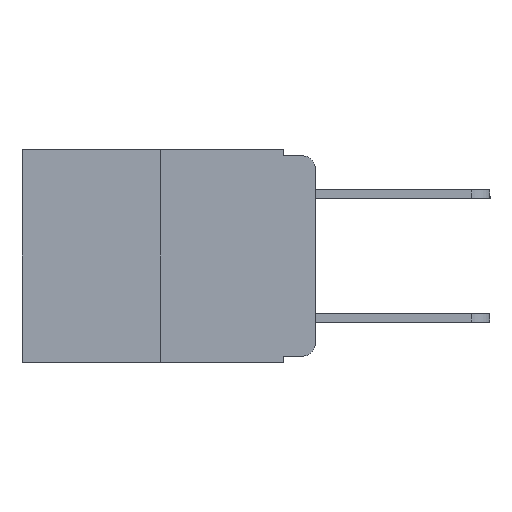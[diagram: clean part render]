
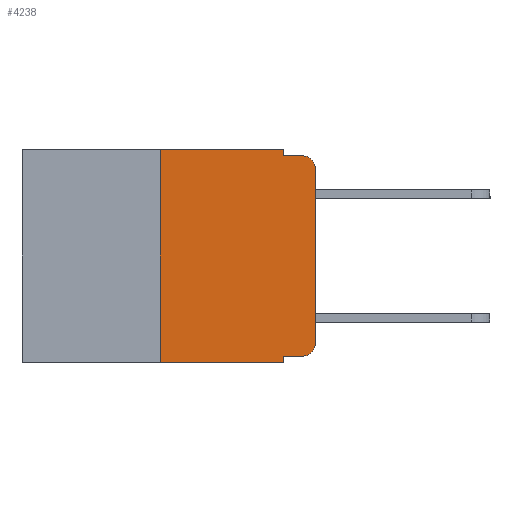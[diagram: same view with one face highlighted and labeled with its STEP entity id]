
A CAD part, left-side view. The second image highlights one B-rep face of the part: STEP entity #4238.
In plain terms, the highlighted planar face has unit normal (-1, 0, 0).
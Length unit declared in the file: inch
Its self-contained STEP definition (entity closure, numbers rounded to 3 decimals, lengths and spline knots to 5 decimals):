
#136 = CIRCLE ( 'NONE', #7155, 0.02 ) ;
#248 = PLANE ( 'NONE',  #5936 ) ;
#509 = EDGE_CURVE ( 'NONE', #4384, #8145, #9554, .T. ) ;
#540 = VECTOR ( 'NONE', #5048, 39.37008 ) ;
#561 = FACE_OUTER_BOUND ( 'NONE', #1097, .T. ) ;
#626 = VERTEX_POINT ( 'NONE', #2970 ) ;
#870 = LINE ( 'NONE', #10910, #10243 ) ;
#949 = DIRECTION ( 'NONE',  ( 0., -1., 0. ) ) ;
#1097 = EDGE_LOOP ( 'NONE', ( #1823, #5097, #2701, #4513, #5716, #2950, #6940, #9742, #6254, #6052 ) ) ;
#1120 = CARTESIAN_POINT ( 'NONE',  ( 0., 0.051, -0.343 ) ) ;
#1334 = EDGE_CURVE ( 'NONE', #10376, #5149, #3584, .T. ) ;
#1509 = DIRECTION ( 'NONE',  ( 1., 0., 0. ) ) ;
#1540 = DIRECTION ( 'NONE',  ( 0., -1., 0. ) ) ;
#1544 = CARTESIAN_POINT ( 'NONE',  ( 0., 0.02, -0.313 ) ) ;
#1609 = VERTEX_POINT ( 'NONE', #5969 ) ;
#1823 = ORIENTED_EDGE ( 'NONE', *, *, #4086, .T. ) ;
#1967 = EDGE_CURVE ( 'NONE', #5149, #4384, #870, .T. ) ;
#2313 = VERTEX_POINT ( 'NONE', #8914 ) ;
#2659 = DIRECTION ( 'NONE',  ( 0., 0., -1. ) ) ;
#2701 = ORIENTED_EDGE ( 'NONE', *, *, #509, .F. ) ;
#2718 = EDGE_CURVE ( 'NONE', #626, #8145, #4612, .T. ) ;
#2926 = CARTESIAN_POINT ( 'NONE',  ( 0., 0.051, -0.01 ) ) ;
#2950 = ORIENTED_EDGE ( 'NONE', *, *, #7742, .F. ) ;
#2970 = CARTESIAN_POINT ( 'NONE',  ( 0., 0., -0.03 ) ) ;
#3584 = LINE ( 'NONE', #8450, #9888 ) ;
#3665 = VECTOR ( 'NONE', #8863, 39.37008 ) ;
#3901 = DIRECTION ( 'NONE',  ( 0., 0., -1. ) ) ;
#4086 = EDGE_CURVE ( 'NONE', #1609, #626, #6971, .T. ) ;
#4238 = ADVANCED_FACE ( 'NONE', ( #561 ), #248, .F. ) ;
#4261 = DIRECTION ( 'NONE',  ( 0., 0., -1. ) ) ;
#4281 = DIRECTION ( 'NONE',  ( -1., 0., 0. ) ) ;
#4311 = CARTESIAN_POINT ( 'NONE',  ( 0., 0.02, -0.03 ) ) ;
#4384 = VERTEX_POINT ( 'NONE', #2926 ) ;
#4513 = ORIENTED_EDGE ( 'NONE', *, *, #1967, .F. ) ;
#4612 = CIRCLE ( 'NONE', #10118, 0.02 ) ;
#4940 = EDGE_CURVE ( 'NONE', #7778, #2313, #5901, .T. ) ;
#5048 = DIRECTION ( 'NONE',  ( 0., -1., 0. ) ) ;
#5096 = CARTESIAN_POINT ( 'NONE',  ( 0., 0.473, -0.343 ) ) ;
#5097 = ORIENTED_EDGE ( 'NONE', *, *, #2718, .T. ) ;
#5149 = VERTEX_POINT ( 'NONE', #10095 ) ;
#5485 = CARTESIAN_POINT ( 'NONE',  ( 0., 0.051, -0.01 ) ) ;
#5499 = VERTEX_POINT ( 'NONE', #1120 ) ;
#5677 = CARTESIAN_POINT ( 'NONE',  ( 0., 0.25, 0. ) ) ;
#5716 = ORIENTED_EDGE ( 'NONE', *, *, #1334, .F. ) ;
#5901 = LINE ( 'NONE', #5909, #540 ) ;
#5909 = CARTESIAN_POINT ( 'NONE',  ( 0., 0.051, -0.333 ) ) ;
#5936 = AXIS2_PLACEMENT_3D ( 'NONE', #7172, #1509, #7199 ) ;
#5969 = CARTESIAN_POINT ( 'NONE',  ( 0., 0., -0.313 ) ) ;
#6000 = DIRECTION ( 'NONE',  ( 0., -1., 0. ) ) ;
#6052 = ORIENTED_EDGE ( 'NONE', *, *, #6123, .T. ) ;
#6123 = EDGE_CURVE ( 'NONE', #2313, #1609, #136, .T. ) ;
#6254 = ORIENTED_EDGE ( 'NONE', *, *, #4940, .T. ) ;
#6361 = VERTEX_POINT ( 'NONE', #7569 ) ;
#6614 = VECTOR ( 'NONE', #9393, 39.37008 ) ;
#6940 = ORIENTED_EDGE ( 'NONE', *, *, #10704, .T. ) ;
#6971 = LINE ( 'NONE', #9817, #9201 ) ;
#7155 = AXIS2_PLACEMENT_3D ( 'NONE', #1544, #7977, #2659 ) ;
#7172 = CARTESIAN_POINT ( 'NONE',  ( 0., 0.473, 0. ) ) ;
#7199 = DIRECTION ( 'NONE',  ( 0., 0., -1. ) ) ;
#7433 = LINE ( 'NONE', #5096, #11164 ) ;
#7569 = CARTESIAN_POINT ( 'NONE',  ( 0., 0.25, -0.343 ) ) ;
#7742 = EDGE_CURVE ( 'NONE', #6361, #10376, #8204, .T. ) ;
#7778 = VERTEX_POINT ( 'NONE', #8891 ) ;
#7977 = DIRECTION ( 'NONE',  ( -1., 0., 0. ) ) ;
#8145 = VERTEX_POINT ( 'NONE', #8460 ) ;
#8204 = LINE ( 'NONE', #5677, #3665 ) ;
#8232 = EDGE_CURVE ( 'NONE', #7778, #5499, #10655, .T. ) ;
#8450 = CARTESIAN_POINT ( 'NONE',  ( 0., 0.473, 0. ) ) ;
#8460 = CARTESIAN_POINT ( 'NONE',  ( 0., 0.02, -0.01 ) ) ;
#8645 = CARTESIAN_POINT ( 'NONE',  ( 0., 0.051, 0. ) ) ;
#8863 = DIRECTION ( 'NONE',  ( 0., 0., 1. ) ) ;
#8891 = CARTESIAN_POINT ( 'NONE',  ( 0., 0.051, -0.333 ) ) ;
#8914 = CARTESIAN_POINT ( 'NONE',  ( 0., 0.02, -0.333 ) ) ;
#9201 = VECTOR ( 'NONE', #9938, 39.37008 ) ;
#9393 = DIRECTION ( 'NONE',  ( 0., 0., -1. ) ) ;
#9554 = LINE ( 'NONE', #5485, #11089 ) ;
#9742 = ORIENTED_EDGE ( 'NONE', *, *, #8232, .F. ) ;
#9817 = CARTESIAN_POINT ( 'NONE',  ( 0., 0., 0. ) ) ;
#9888 = VECTOR ( 'NONE', #1540, 39.37008 ) ;
#9938 = DIRECTION ( 'NONE',  ( 0., 0., 1. ) ) ;
#10095 = CARTESIAN_POINT ( 'NONE',  ( 0., 0.051, 0. ) ) ;
#10118 = AXIS2_PLACEMENT_3D ( 'NONE', #4311, #4281, #4261 ) ;
#10243 = VECTOR ( 'NONE', #3901, 39.37008 ) ;
#10376 = VERTEX_POINT ( 'NONE', #11038 ) ;
#10655 = LINE ( 'NONE', #8645, #6614 ) ;
#10704 = EDGE_CURVE ( 'NONE', #6361, #5499, #7433, .T. ) ;
#10910 = CARTESIAN_POINT ( 'NONE',  ( 0., 0.051, 0. ) ) ;
#11038 = CARTESIAN_POINT ( 'NONE',  ( 0., 0.25, 0. ) ) ;
#11089 = VECTOR ( 'NONE', #949, 39.37008 ) ;
#11164 = VECTOR ( 'NONE', #6000, 39.37008 ) ;
